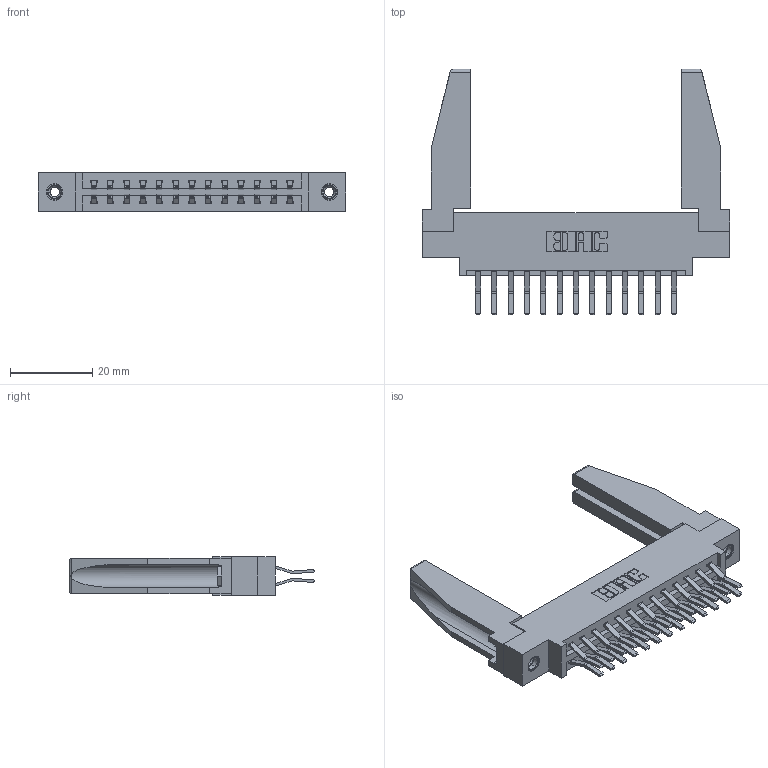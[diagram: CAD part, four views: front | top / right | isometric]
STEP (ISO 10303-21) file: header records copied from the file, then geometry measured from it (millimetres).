
FILE_DESCRIPTION (( 'STEP AP203' ), '1' );
FILE_NAME ('337-026-560-878.STEP', '2019-10-10T22:19:47', ( '' ), ( '' ), 'SwSTEP 2.0', 'SolidWorks 2016', '' );
FILE_SCHEMA (( 'CONFIG_CONTROL_DESIGN' ));
Length unit declared in the file: inch
Products named in the file (5): 337 Part_0.170 Offset - 0.156 Dia-TI; 345-250-001_345-250-001-102; 345-292-001_560 Tail; 337-026-560-878; 307-220-078
Assembly tree (31 placements, depth 2):
  337-026-560-878
    337 Part_0.170 Offset - 0.156 Dia-TI
    345-292-001_560 Tail  x26
    345-250-001_345-250-001-102  x2
    307-220-078  x2
Bounding box: 74.52 x 59.58 x 9.4 mm (x, y, z)
Volume: 11514.1 mm3; surface area: 12652.1 mm2
Topology: 31 solids, 31 shells, 1704 faces, 4995 edges, 3286 vertices
Faces by surface type: plane 1146, cylinder 542, cone 12, torus 4
Entity records: 16490 total; most frequent: CARTESIAN_POINT 2804, ORIENTED_EDGE 2696, DIRECTION 2448, EDGE_CURVE 1348, LINE 1178, VECTOR 1178, VERTEX_POINT 892, AXIS2_PLACEMENT_3D 635
